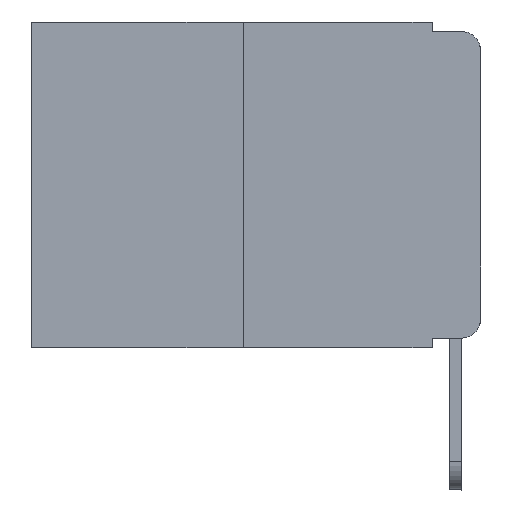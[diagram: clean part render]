
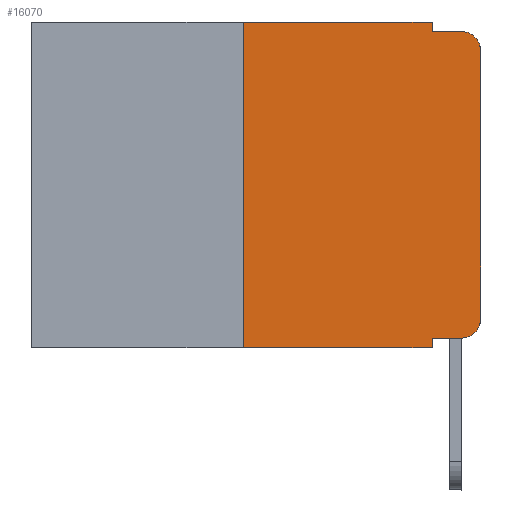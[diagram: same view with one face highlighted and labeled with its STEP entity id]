
A CAD part, left-side view. The second image highlights one B-rep face of the part: STEP entity #16070.
In plain terms, the highlighted planar face has unit normal (-1, 0, 0).
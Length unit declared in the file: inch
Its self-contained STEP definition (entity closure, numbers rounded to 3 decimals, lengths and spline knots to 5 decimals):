
#393 = EDGE_CURVE ( 'NONE', #20343, #3521, #22531, .T. ) ;
#1044 = CARTESIAN_POINT ( 'NONE',  ( 0., 0.25, -0.343 ) ) ;
#1366 = DIRECTION ( 'NONE',  ( 0., 0., 1. ) ) ;
#1893 = CARTESIAN_POINT ( 'NONE',  ( 0., 0.051, 0. ) ) ;
#2557 = DIRECTION ( 'NONE',  ( 1., 0., 0. ) ) ;
#2601 = VERTEX_POINT ( 'NONE', #13355 ) ;
#2656 = DIRECTION ( 'NONE',  ( 0., -1., 0. ) ) ;
#2859 = DIRECTION ( 'NONE',  ( 0., 0., -1. ) ) ;
#2988 = VERTEX_POINT ( 'NONE', #14292 ) ;
#3213 = VECTOR ( 'NONE', #14733, 39.37008 ) ;
#3521 = VERTEX_POINT ( 'NONE', #4328 ) ;
#3728 = ORIENTED_EDGE ( 'NONE', *, *, #19704, .T. ) ;
#4328 = CARTESIAN_POINT ( 'NONE',  ( 0., 0.051, -0.343 ) ) ;
#4478 = VECTOR ( 'NONE', #5332, 39.37008 ) ;
#4890 = CARTESIAN_POINT ( 'NONE',  ( 0., 0.02, -0.03 ) ) ;
#5274 = VECTOR ( 'NONE', #2656, 39.37008 ) ;
#5332 = DIRECTION ( 'NONE',  ( 0., 0., 1. ) ) ;
#5447 = CARTESIAN_POINT ( 'NONE',  ( 0., 0., 0. ) ) ;
#6271 = CARTESIAN_POINT ( 'NONE',  ( 0., 0.473, 0. ) ) ;
#6894 = AXIS2_PLACEMENT_3D ( 'NONE', #13509, #2557, #15423 ) ;
#7421 = EDGE_CURVE ( 'NONE', #9365, #14968, #19889, .T. ) ;
#7820 = LINE ( 'NONE', #18785, #10342 ) ;
#7847 = CARTESIAN_POINT ( 'NONE',  ( 0., 0.473, -0.343 ) ) ;
#8423 = FACE_OUTER_BOUND ( 'NONE', #15464, .T. ) ;
#8778 = ORIENTED_EDGE ( 'NONE', *, *, #7421, .T. ) ;
#8838 = LINE ( 'NONE', #13913, #14129 ) ;
#8996 = CIRCLE ( 'NONE', #11688, 0.02 ) ;
#9365 = VERTEX_POINT ( 'NONE', #12516 ) ;
#9668 = EDGE_CURVE ( 'NONE', #12578, #3521, #23769, .T. ) ;
#9890 = ORIENTED_EDGE ( 'NONE', *, *, #11731, .F. ) ;
#10100 = VECTOR ( 'NONE', #21618, 39.37008 ) ;
#10342 = VECTOR ( 'NONE', #13258, 39.37008 ) ;
#10631 = ORIENTED_EDGE ( 'NONE', *, *, #19929, .F. ) ;
#11688 = AXIS2_PLACEMENT_3D ( 'NONE', #4890, #14288, #14536 ) ;
#11731 = EDGE_CURVE ( 'NONE', #20343, #22658, #16496, .T. ) ;
#11881 = VERTEX_POINT ( 'NONE', #17098 ) ;
#12211 = ORIENTED_EDGE ( 'NONE', *, *, #13322, .F. ) ;
#12240 = CARTESIAN_POINT ( 'NONE',  ( 0., 0.051, -0.333 ) ) ;
#12516 = CARTESIAN_POINT ( 'NONE',  ( 0., 0.02, -0.333 ) ) ;
#12578 = VERTEX_POINT ( 'NONE', #12240 ) ;
#12641 = EDGE_CURVE ( 'NONE', #11881, #2988, #8996, .T. ) ;
#12660 = CARTESIAN_POINT ( 'NONE',  ( 0., 0.25, 0. ) ) ;
#13097 = CARTESIAN_POINT ( 'NONE',  ( 0., 0., -0.313 ) ) ;
#13258 = DIRECTION ( 'NONE',  ( 0., -1., 0. ) ) ;
#13322 = EDGE_CURVE ( 'NONE', #20340, #2988, #7820, .T. ) ;
#13355 = CARTESIAN_POINT ( 'NONE',  ( 0., 0.051, 0. ) ) ;
#13509 = CARTESIAN_POINT ( 'NONE',  ( 0., 0.473, 0. ) ) ;
#13913 = CARTESIAN_POINT ( 'NONE',  ( 0., 0.051, -0.333 ) ) ;
#14129 = VECTOR ( 'NONE', #23174, 39.37008 ) ;
#14288 = DIRECTION ( 'NONE',  ( -1., 0., 0. ) ) ;
#14292 = CARTESIAN_POINT ( 'NONE',  ( 0., 0.02, -0.01 ) ) ;
#14536 = DIRECTION ( 'NONE',  ( 0., 0., -1. ) ) ;
#14733 = DIRECTION ( 'NONE',  ( 0., -1., 0. ) ) ;
#14968 = VERTEX_POINT ( 'NONE', #13097 ) ;
#15174 = ORIENTED_EDGE ( 'NONE', *, *, #20429, .T. ) ;
#15423 = DIRECTION ( 'NONE',  ( 0., 0., -1. ) ) ;
#15464 = EDGE_LOOP ( 'NONE', ( #3728, #21085, #12211, #21789, #10631, #9890, #19870, #21595, #15174, #8778 ) ) ;
#15845 = CARTESIAN_POINT ( 'NONE',  ( 0., 0.02, -0.313 ) ) ;
#16070 = ADVANCED_FACE ( 'NONE', ( #8423 ), #17332, .F. ) ;
#16496 = LINE ( 'NONE', #12660, #22094 ) ;
#16519 = LINE ( 'NONE', #5447, #4478 ) ;
#16685 = LINE ( 'NONE', #1893, #23297 ) ;
#17098 = CARTESIAN_POINT ( 'NONE',  ( 0., 0., -0.03 ) ) ;
#17332 = PLANE ( 'NONE',  #6894 ) ;
#17892 = CARTESIAN_POINT ( 'NONE',  ( 0., 0.051, -0.01 ) ) ;
#18373 = CARTESIAN_POINT ( 'NONE',  ( 0., 0.051, 0. ) ) ;
#18785 = CARTESIAN_POINT ( 'NONE',  ( 0., 0.051, -0.01 ) ) ;
#19265 = LINE ( 'NONE', #6271, #5274 ) ;
#19276 = EDGE_CURVE ( 'NONE', #2601, #20340, #16685, .T. ) ;
#19704 = EDGE_CURVE ( 'NONE', #14968, #11881, #16519, .T. ) ;
#19870 = ORIENTED_EDGE ( 'NONE', *, *, #393, .T. ) ;
#19889 = CIRCLE ( 'NONE', #22940, 0.02 ) ;
#19929 = EDGE_CURVE ( 'NONE', #22658, #2601, #19265, .T. ) ;
#20340 = VERTEX_POINT ( 'NONE', #17892 ) ;
#20343 = VERTEX_POINT ( 'NONE', #1044 ) ;
#20398 = DIRECTION ( 'NONE',  ( 0., 0., -1. ) ) ;
#20429 = EDGE_CURVE ( 'NONE', #12578, #9365, #8838, .T. ) ;
#21085 = ORIENTED_EDGE ( 'NONE', *, *, #12641, .T. ) ;
#21595 = ORIENTED_EDGE ( 'NONE', *, *, #9668, .F. ) ;
#21618 = DIRECTION ( 'NONE',  ( 0., 0., -1. ) ) ;
#21789 = ORIENTED_EDGE ( 'NONE', *, *, #19276, .F. ) ;
#22094 = VECTOR ( 'NONE', #1366, 39.37008 ) ;
#22531 = LINE ( 'NONE', #7847, #3213 ) ;
#22658 = VERTEX_POINT ( 'NONE', #23126 ) ;
#22940 = AXIS2_PLACEMENT_3D ( 'NONE', #15845, #23190, #2859 ) ;
#23126 = CARTESIAN_POINT ( 'NONE',  ( 0., 0.25, 0. ) ) ;
#23174 = DIRECTION ( 'NONE',  ( 0., -1., 0. ) ) ;
#23190 = DIRECTION ( 'NONE',  ( -1., 0., 0. ) ) ;
#23297 = VECTOR ( 'NONE', #20398, 39.37008 ) ;
#23769 = LINE ( 'NONE', #18373, #10100 ) ;
